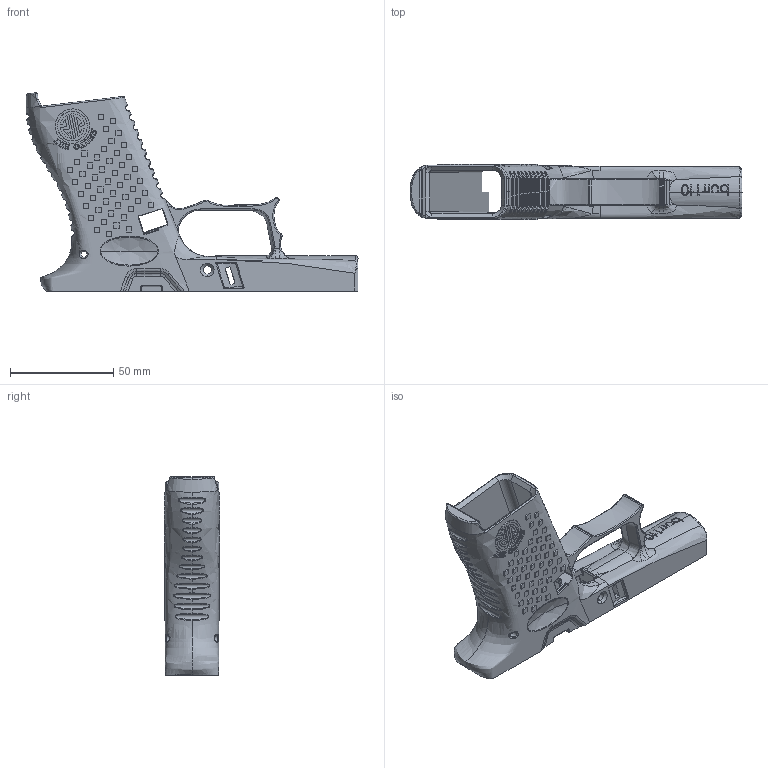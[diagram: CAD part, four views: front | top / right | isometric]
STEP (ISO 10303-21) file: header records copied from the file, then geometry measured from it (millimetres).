
FILE_DESCRIPTION (( 'STEP AP203' ), '1' );
FILE_NAME ('43X SideLogo FDM.STEP', '2020-12-17T01:04:10', ( '' ), ( '' ), 'SwSTEP 2.0', 'SolidWorks 2016', '' );
FILE_SCHEMA (( 'CONFIG_CONTROL_DESIGN' ));
Products named in the file (1): 43X SideLogo FDM
Bounding box: 160.56 x 26.9 x 95.92 mm (x, y, z)
Volume: 63916.5 mm3; surface area: 39077.3 mm2
Topology: 1 solids, 1 shells, 2209 faces, 5924 edges, 3805 vertices
Faces by surface type: plane 1142, bspline 640, cylinder 387, torus 26, cone 12, sphere 2
Entity records: 395436 total; most frequent: CARTESIAN_POINT 349455, ORIENTED_EDGE 11776, DIRECTION 5959, EDGE_CURVE 5888, VERTEX_POINT 3805, B_SPLINE_CURVE_WITH_KNOTS 3466, EDGE_LOOP 2355, FACE_OUTER_BOUND 2209
